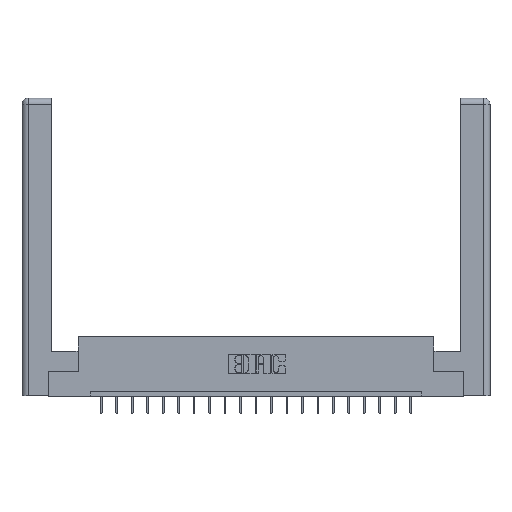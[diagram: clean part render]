
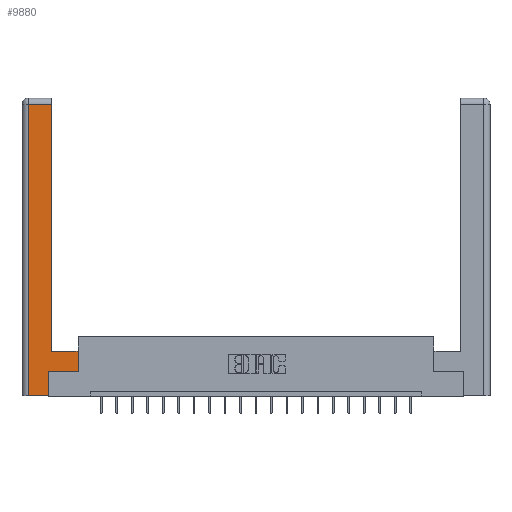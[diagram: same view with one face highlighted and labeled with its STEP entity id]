
A CAD part, top view. The second image highlights one B-rep face of the part: STEP entity #9880.
In plain terms, the highlighted planar face has unit normal (0, 0, 1).
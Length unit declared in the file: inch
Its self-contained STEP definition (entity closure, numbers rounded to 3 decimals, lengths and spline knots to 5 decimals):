
#27 = DIRECTION ( 'NONE',  ( 0., 1., 0. ) ) ;
#174 = ORIENTED_EDGE ( 'NONE', *, *, #13687, .T. ) ;
#448 = LINE ( 'NONE', #16725, #14929 ) ;
#564 = CARTESIAN_POINT ( 'NONE',  ( 0.295, 0.45, 0. ) ) ;
#836 = CARTESIAN_POINT ( 'NONE',  ( 0.565, 0.45, 0. ) ) ;
#989 = EDGE_CURVE ( 'NONE', #19196, #16824, #9161, .T. ) ;
#2075 = LINE ( 'NONE', #11413, #19871 ) ;
#2320 = DIRECTION ( 'NONE',  ( 0., 1., 0. ) ) ;
#2637 = EDGE_CURVE ( 'NONE', #16824, #13204, #448, .T. ) ;
#3052 = VERTEX_POINT ( 'NONE', #5190 ) ;
#3764 = CARTESIAN_POINT ( 'NONE',  ( 0.295, 2.94, 0. ) ) ;
#3832 = VERTEX_POINT ( 'NONE', #13531 ) ;
#4265 = EDGE_LOOP ( 'NONE', ( #5014, #18009, #9154, #16355, #174, #7630, #6281, #10779 ) ) ;
#4553 = VERTEX_POINT ( 'NONE', #19580 ) ;
#4573 = VERTEX_POINT ( 'NONE', #17810 ) ;
#4962 = CARTESIAN_POINT ( 'NONE',  ( 0., 0., 0. ) ) ;
#5014 = ORIENTED_EDGE ( 'NONE', *, *, #2637, .T. ) ;
#5190 = CARTESIAN_POINT ( 'NONE',  ( 0.265, 0.245, 0. ) ) ;
#5284 = VECTOR ( 'NONE', #5453, 39.37008 ) ;
#5453 = DIRECTION ( 'NONE',  ( 1., 0., 0. ) ) ;
#6281 = ORIENTED_EDGE ( 'NONE', *, *, #17472, .T. ) ;
#6465 = AXIS2_PLACEMENT_3D ( 'NONE', #4962, #16746, #18115 ) ;
#7069 = LINE ( 'NONE', #15328, #5284 ) ;
#7114 = LINE ( 'NONE', #8048, #17046 ) ;
#7630 = ORIENTED_EDGE ( 'NONE', *, *, #15436, .T. ) ;
#8048 = CARTESIAN_POINT ( 'NONE',  ( 0.265, 0.245, 0. ) ) ;
#8273 = CARTESIAN_POINT ( 'NONE',  ( 0.565, 0.45, 0. ) ) ;
#8805 = VECTOR ( 'NONE', #16181, 39.37008 ) ;
#9154 = ORIENTED_EDGE ( 'NONE', *, *, #15955, .T. ) ;
#9161 = LINE ( 'NONE', #564, #9409 ) ;
#9409 = VECTOR ( 'NONE', #11991, 39.37008 ) ;
#9880 = ADVANCED_FACE ( 'NONE', ( #17732 ), #13061, .F. ) ;
#9904 = DIRECTION ( 'NONE',  ( 0., 1., 0. ) ) ;
#10279 = CARTESIAN_POINT ( 'NONE',  ( 0.265, 0., 0. ) ) ;
#10779 = ORIENTED_EDGE ( 'NONE', *, *, #989, .T. ) ;
#11413 = CARTESIAN_POINT ( 'NONE',  ( 0.0615, 2.94, 0. ) ) ;
#11991 = DIRECTION ( 'NONE',  ( -1., 0., 0. ) ) ;
#13061 = PLANE ( 'NONE',  #6465 ) ;
#13204 = VERTEX_POINT ( 'NONE', #3764 ) ;
#13531 = CARTESIAN_POINT ( 'NONE',  ( 0.565, 0.245, 0. ) ) ;
#13687 = EDGE_CURVE ( 'NONE', #15708, #3052, #7114, .T. ) ;
#14166 = LINE ( 'NONE', #20938, #8805 ) ;
#14929 = VECTOR ( 'NONE', #9904, 39.37008 ) ;
#15133 = CARTESIAN_POINT ( 'NONE',  ( 0.295, 0.45, 0. ) ) ;
#15323 = LINE ( 'NONE', #836, #16085 ) ;
#15328 = CARTESIAN_POINT ( 'NONE',  ( 0.265, 0., 0. ) ) ;
#15401 = LINE ( 'NONE', #16017, #19961 ) ;
#15436 = EDGE_CURVE ( 'NONE', #3052, #3832, #14166, .T. ) ;
#15708 = VERTEX_POINT ( 'NONE', #10279 ) ;
#15955 = EDGE_CURVE ( 'NONE', #4573, #4553, #15401, .T. ) ;
#16017 = CARTESIAN_POINT ( 'NONE',  ( 0.0615, 0., 0. ) ) ;
#16085 = VECTOR ( 'NONE', #2320, 39.37008 ) ;
#16181 = DIRECTION ( 'NONE',  ( 1., 0., 0. ) ) ;
#16355 = ORIENTED_EDGE ( 'NONE', *, *, #16385, .T. ) ;
#16385 = EDGE_CURVE ( 'NONE', #4553, #15708, #7069, .T. ) ;
#16522 = DIRECTION ( 'NONE',  ( -1., 0., 0. ) ) ;
#16725 = CARTESIAN_POINT ( 'NONE',  ( 0.295, 3., 0. ) ) ;
#16746 = DIRECTION ( 'NONE',  ( 0., 0., -1. ) ) ;
#16824 = VERTEX_POINT ( 'NONE', #15133 ) ;
#17046 = VECTOR ( 'NONE', #27, 39.37008 ) ;
#17472 = EDGE_CURVE ( 'NONE', #3832, #19196, #15323, .T. ) ;
#17732 = FACE_OUTER_BOUND ( 'NONE', #4265, .T. ) ;
#17810 = CARTESIAN_POINT ( 'NONE',  ( 0.0615, 2.94, 0. ) ) ;
#17929 = EDGE_CURVE ( 'NONE', #13204, #4573, #2075, .T. ) ;
#18009 = ORIENTED_EDGE ( 'NONE', *, *, #17929, .T. ) ;
#18115 = DIRECTION ( 'NONE',  ( -1., 0., 0. ) ) ;
#19196 = VERTEX_POINT ( 'NONE', #8273 ) ;
#19286 = DIRECTION ( 'NONE',  ( 0., -1., 0. ) ) ;
#19580 = CARTESIAN_POINT ( 'NONE',  ( 0.0615, 0., 0. ) ) ;
#19871 = VECTOR ( 'NONE', #16522, 39.37008 ) ;
#19961 = VECTOR ( 'NONE', #19286, 39.37008 ) ;
#20938 = CARTESIAN_POINT ( 'NONE',  ( 0.565, 0.245, 0. ) ) ;
